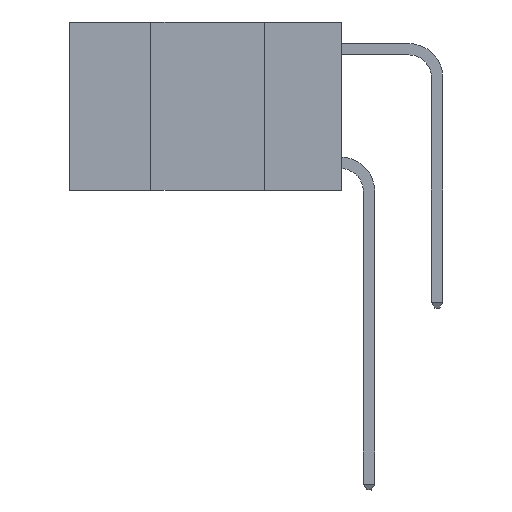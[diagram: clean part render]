
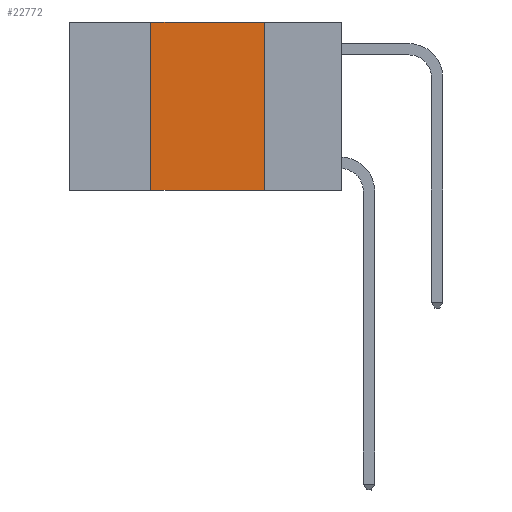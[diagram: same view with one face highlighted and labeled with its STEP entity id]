
A CAD part, left-side view. The second image highlights one B-rep face of the part: STEP entity #22772.
In plain terms, the highlighted planar face has unit normal (-1, 0, 0).
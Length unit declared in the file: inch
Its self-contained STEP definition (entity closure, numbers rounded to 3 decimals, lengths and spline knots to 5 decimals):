
#811 = VECTOR ( 'NONE', #12602, 39.37008 ) ;
#1143 = LINE ( 'NONE', #5665, #14673 ) ;
#1679 = CARTESIAN_POINT ( 'NONE',  ( 0., 0.42, 0. ) ) ;
#2274 = ORIENTED_EDGE ( 'NONE', *, *, #27978, .F. ) ;
#3730 = LINE ( 'NONE', #1679, #811 ) ;
#4404 = AXIS2_PLACEMENT_3D ( 'NONE', #20173, #15823, #16263 ) ;
#4476 = EDGE_CURVE ( 'NONE', #17696, #14251, #23004, .T. ) ;
#4875 = VECTOR ( 'NONE', #15927, 39.37008 ) ;
#5665 = CARTESIAN_POINT ( 'NONE',  ( 0., 0.6, -0.37 ) ) ;
#6652 = CARTESIAN_POINT ( 'NONE',  ( 0., 0.42, 0. ) ) ;
#6953 = FACE_OUTER_BOUND ( 'NONE', #9977, .T. ) ;
#7063 = CARTESIAN_POINT ( 'NONE',  ( 0., 0.17, 0. ) ) ;
#8039 = ORIENTED_EDGE ( 'NONE', *, *, #4476, .F. ) ;
#8580 = ORIENTED_EDGE ( 'NONE', *, *, #9274, .F. ) ;
#9228 = CARTESIAN_POINT ( 'NONE',  ( 0., 0.17, -0.37 ) ) ;
#9274 = EDGE_CURVE ( 'NONE', #14251, #28253, #17970, .T. ) ;
#9977 = EDGE_LOOP ( 'NONE', ( #8580, #8039, #2274, #25274 ) ) ;
#10505 = EDGE_CURVE ( 'NONE', #21437, #28253, #1143, .T. ) ;
#10517 = VECTOR ( 'NONE', #25492, 39.37008 ) ;
#11304 = PLANE ( 'NONE',  #4404 ) ;
#12602 = DIRECTION ( 'NONE',  ( 0., 0., 1. ) ) ;
#14251 = VERTEX_POINT ( 'NONE', #27896 ) ;
#14673 = VECTOR ( 'NONE', #23391, 39.37008 ) ;
#15823 = DIRECTION ( 'NONE',  ( 1., 0., 0. ) ) ;
#15927 = DIRECTION ( 'NONE',  ( 0., 0., -1. ) ) ;
#16263 = DIRECTION ( 'NONE',  ( 0., 0., -1. ) ) ;
#17696 = VERTEX_POINT ( 'NONE', #6652 ) ;
#17970 = LINE ( 'NONE', #7063, #4875 ) ;
#18537 = CARTESIAN_POINT ( 'NONE',  ( 0., 0.42, -0.37 ) ) ;
#20173 = CARTESIAN_POINT ( 'NONE',  ( 0., 0.6, 0. ) ) ;
#21437 = VERTEX_POINT ( 'NONE', #18537 ) ;
#22772 = ADVANCED_FACE ( 'NONE', ( #6953 ), #11304, .F. ) ;
#23004 = LINE ( 'NONE', #27087, #10517 ) ;
#23391 = DIRECTION ( 'NONE',  ( 0., -1., 0. ) ) ;
#25274 = ORIENTED_EDGE ( 'NONE', *, *, #10505, .T. ) ;
#25492 = DIRECTION ( 'NONE',  ( 0., -1., 0. ) ) ;
#27087 = CARTESIAN_POINT ( 'NONE',  ( 0., 0.6, 0. ) ) ;
#27896 = CARTESIAN_POINT ( 'NONE',  ( 0., 0.17, 0. ) ) ;
#27978 = EDGE_CURVE ( 'NONE', #21437, #17696, #3730, .T. ) ;
#28253 = VERTEX_POINT ( 'NONE', #9228 ) ;
